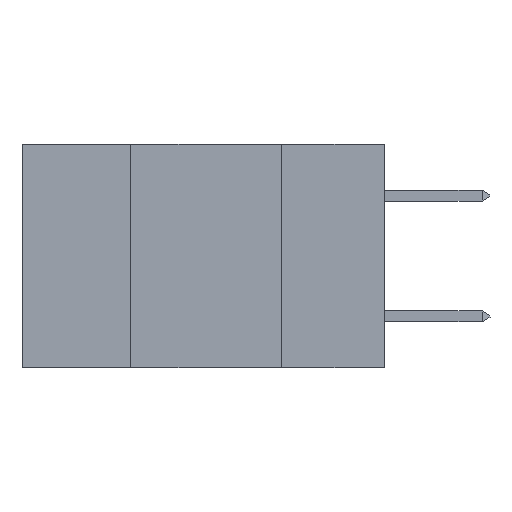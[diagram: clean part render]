
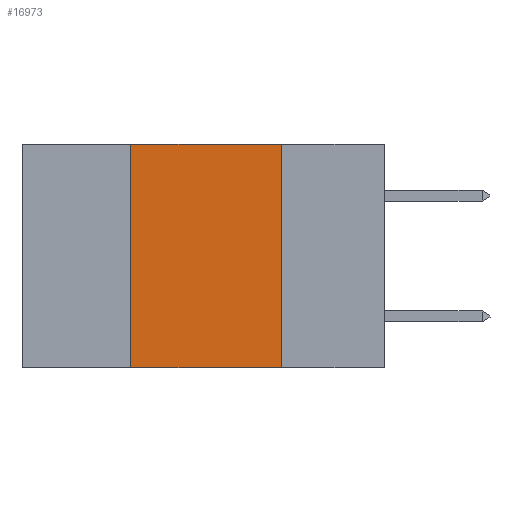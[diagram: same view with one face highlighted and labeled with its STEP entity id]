
A CAD part, left-side view. The second image highlights one B-rep face of the part: STEP entity #16973.
In plain terms, the highlighted planar face has unit normal (-1, 0, 0).
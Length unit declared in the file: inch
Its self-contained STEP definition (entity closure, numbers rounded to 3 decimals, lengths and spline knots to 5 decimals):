
#958 = VERTEX_POINT ( 'NONE', #11935 ) ;
#1314 = EDGE_LOOP ( 'NONE', ( #5759, #4164, #15780, #15240 ) ) ;
#1390 = DIRECTION ( 'NONE',  ( 1., 0., 0. ) ) ;
#2198 = CARTESIAN_POINT ( 'NONE',  ( 0., 0.17, -0.37 ) ) ;
#2422 = CARTESIAN_POINT ( 'NONE',  ( 0., 0.17, 0. ) ) ;
#2753 = VECTOR ( 'NONE', #15938, 39.37008 ) ;
#4164 = ORIENTED_EDGE ( 'NONE', *, *, #12243, .F. ) ;
#4811 = EDGE_CURVE ( 'NONE', #11716, #8697, #8156, .T. ) ;
#5281 = VECTOR ( 'NONE', #7889, 39.37008 ) ;
#5464 = CARTESIAN_POINT ( 'NONE',  ( 0., 0.17, 0. ) ) ;
#5759 = ORIENTED_EDGE ( 'NONE', *, *, #4811, .F. ) ;
#5801 = LINE ( 'NONE', #6311, #5281 ) ;
#6311 = CARTESIAN_POINT ( 'NONE',  ( 0., 0.42, 0. ) ) ;
#7668 = LINE ( 'NONE', #9168, #15914 ) ;
#7889 = DIRECTION ( 'NONE',  ( 0., 0., 1. ) ) ;
#8156 = LINE ( 'NONE', #2422, #11944 ) ;
#8697 = VERTEX_POINT ( 'NONE', #2198 ) ;
#9168 = CARTESIAN_POINT ( 'NONE',  ( 0., 0.6, -0.37 ) ) ;
#9642 = CARTESIAN_POINT ( 'NONE',  ( 0., 0.6, 0. ) ) ;
#11424 = EDGE_CURVE ( 'NONE', #958, #12395, #5801, .T. ) ;
#11716 = VERTEX_POINT ( 'NONE', #5464 ) ;
#11935 = CARTESIAN_POINT ( 'NONE',  ( 0., 0.42, -0.37 ) ) ;
#11944 = VECTOR ( 'NONE', #17016, 39.37008 ) ;
#12243 = EDGE_CURVE ( 'NONE', #12395, #11716, #15721, .T. ) ;
#12395 = VERTEX_POINT ( 'NONE', #13160 ) ;
#12903 = DIRECTION ( 'NONE',  ( 0., 0., -1. ) ) ;
#13160 = CARTESIAN_POINT ( 'NONE',  ( 0., 0.42, 0. ) ) ;
#13922 = EDGE_CURVE ( 'NONE', #958, #8697, #7668, .T. ) ;
#14203 = AXIS2_PLACEMENT_3D ( 'NONE', #9642, #1390, #12903 ) ;
#15240 = ORIENTED_EDGE ( 'NONE', *, *, #13922, .T. ) ;
#15721 = LINE ( 'NONE', #20569, #2753 ) ;
#15780 = ORIENTED_EDGE ( 'NONE', *, *, #11424, .F. ) ;
#15914 = VECTOR ( 'NONE', #18588, 39.37008 ) ;
#15938 = DIRECTION ( 'NONE',  ( 0., -1., 0. ) ) ;
#16973 = ADVANCED_FACE ( 'NONE', ( #19470 ), #20628, .F. ) ;
#17016 = DIRECTION ( 'NONE',  ( 0., 0., -1. ) ) ;
#18588 = DIRECTION ( 'NONE',  ( 0., -1., 0. ) ) ;
#19470 = FACE_OUTER_BOUND ( 'NONE', #1314, .T. ) ;
#20569 = CARTESIAN_POINT ( 'NONE',  ( 0., 0.6, 0. ) ) ;
#20628 = PLANE ( 'NONE',  #14203 ) ;
